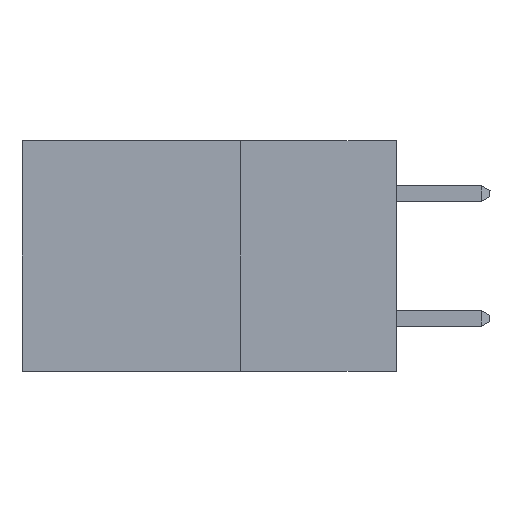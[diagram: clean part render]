
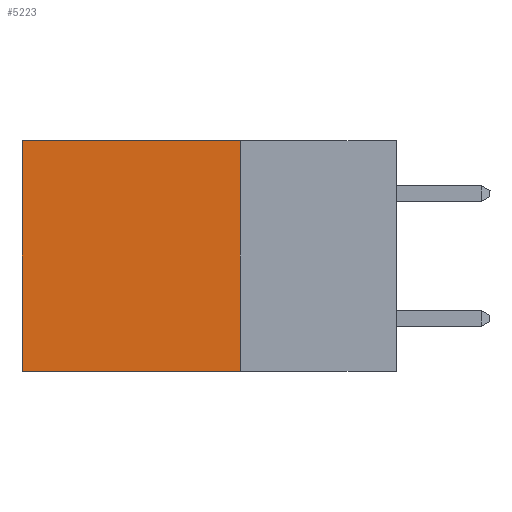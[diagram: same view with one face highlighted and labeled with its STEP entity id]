
A CAD part, left-side view. The second image highlights one B-rep face of the part: STEP entity #5223.
In plain terms, the highlighted planar face has unit normal (-1, 0, 0).
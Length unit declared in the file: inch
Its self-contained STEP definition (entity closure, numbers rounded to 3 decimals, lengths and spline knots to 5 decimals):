
#1241 = DIRECTION ( 'NONE',  ( 1., 0., 0. ) ) ;
#2103 = LINE ( 'NONE', #8436, #13177 ) ;
#2455 = VERTEX_POINT ( 'NONE', #8981 ) ;
#2495 = VECTOR ( 'NONE', #9648, 39.37008 ) ;
#2529 = EDGE_CURVE ( 'NONE', #6422, #2455, #3550, .T. ) ;
#3358 = EDGE_CURVE ( 'NONE', #10788, #6422, #6791, .T. ) ;
#3550 = LINE ( 'NONE', #6584, #9057 ) ;
#4165 = ORIENTED_EDGE ( 'NONE', *, *, #4411, .F. ) ;
#4183 = FACE_OUTER_BOUND ( 'NONE', #5047, .T. ) ;
#4411 = EDGE_CURVE ( 'NONE', #12065, #2455, #2103, .T. ) ;
#5047 = EDGE_LOOP ( 'NONE', ( #6686, #4165, #12694, #7428 ) ) ;
#5223 = ADVANCED_FACE ( 'NONE', ( #4183 ), #7881, .F. ) ;
#5952 = CARTESIAN_POINT ( 'NONE',  ( 0.298, 0.25, 0. ) ) ;
#6422 = VERTEX_POINT ( 'NONE', #11032 ) ;
#6440 = VECTOR ( 'NONE', #11235, 39.37008 ) ;
#6445 = LINE ( 'NONE', #12952, #2495 ) ;
#6584 = CARTESIAN_POINT ( 'NONE',  ( 0.298, 0.6, 0. ) ) ;
#6686 = ORIENTED_EDGE ( 'NONE', *, *, #2529, .T. ) ;
#6791 = LINE ( 'NONE', #10726, #6440 ) ;
#7428 = ORIENTED_EDGE ( 'NONE', *, *, #3358, .T. ) ;
#7881 = PLANE ( 'NONE',  #8322 ) ;
#8322 = AXIS2_PLACEMENT_3D ( 'NONE', #12311, #1241, #8990 ) ;
#8380 = CARTESIAN_POINT ( 'NONE',  ( 0.298, 0.25, -0.37 ) ) ;
#8436 = CARTESIAN_POINT ( 'NONE',  ( 0.298, 0.25, -0.37 ) ) ;
#8981 = CARTESIAN_POINT ( 'NONE',  ( 0.298, 0.6, -0.37 ) ) ;
#8990 = DIRECTION ( 'NONE',  ( 0., 0., -1. ) ) ;
#9057 = VECTOR ( 'NONE', #13213, 39.37008 ) ;
#9648 = DIRECTION ( 'NONE',  ( 0., 0., -1. ) ) ;
#10726 = CARTESIAN_POINT ( 'NONE',  ( 0.298, 0.25, 0. ) ) ;
#10788 = VERTEX_POINT ( 'NONE', #5952 ) ;
#11004 = EDGE_CURVE ( 'NONE', #10788, #12065, #6445, .T. ) ;
#11032 = CARTESIAN_POINT ( 'NONE',  ( 0.298, 0.6, 0. ) ) ;
#11235 = DIRECTION ( 'NONE',  ( 0., 1., 0. ) ) ;
#12065 = VERTEX_POINT ( 'NONE', #8380 ) ;
#12311 = CARTESIAN_POINT ( 'NONE',  ( 0.298, 0.25, 0. ) ) ;
#12694 = ORIENTED_EDGE ( 'NONE', *, *, #11004, .F. ) ;
#12725 = DIRECTION ( 'NONE',  ( 0., 1., 0. ) ) ;
#12952 = CARTESIAN_POINT ( 'NONE',  ( 0.298, 0.25, 0. ) ) ;
#13177 = VECTOR ( 'NONE', #12725, 39.37008 ) ;
#13213 = DIRECTION ( 'NONE',  ( 0., 0., -1. ) ) ;
